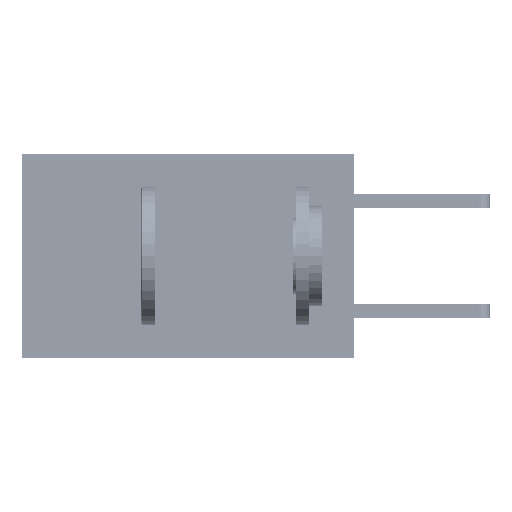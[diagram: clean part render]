
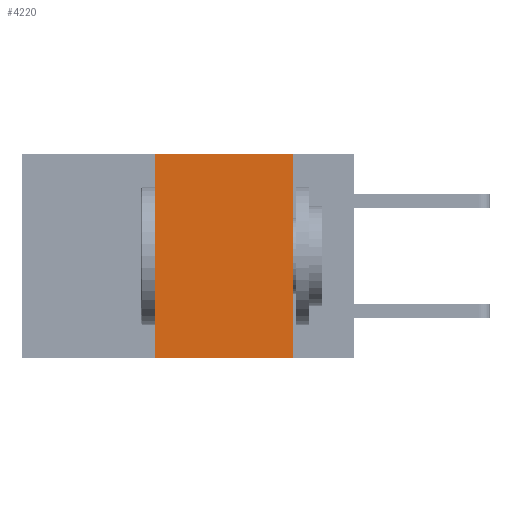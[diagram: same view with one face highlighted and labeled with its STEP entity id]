
A CAD part, left-side view. The second image highlights one B-rep face of the part: STEP entity #4220.
In plain terms, the highlighted planar face has unit normal (-1, 0, 0).
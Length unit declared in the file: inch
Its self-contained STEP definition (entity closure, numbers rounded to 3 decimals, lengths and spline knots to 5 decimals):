
#1895 = ORIENTED_EDGE ( 'NONE', *, *, #33448, .T. ) ;
#1991 = CARTESIAN_POINT ( 'NONE',  ( 0., 0.36, -0.37 ) ) ;
#4220 = ADVANCED_FACE ( 'NONE', ( #29030 ), #33040, .F. ) ;
#5551 = CARTESIAN_POINT ( 'NONE',  ( 0., 0.11, 0. ) ) ;
#6119 = DIRECTION ( 'NONE',  ( 0., -1., 0. ) ) ;
#8300 = CARTESIAN_POINT ( 'NONE',  ( 0., 0.6, 0. ) ) ;
#8950 = CARTESIAN_POINT ( 'NONE',  ( 0., 0.11, -0.37 ) ) ;
#9851 = DIRECTION ( 'NONE',  ( 1., 0., 0. ) ) ;
#11675 = CARTESIAN_POINT ( 'NONE',  ( 0., 0.6, -0.37 ) ) ;
#13910 = DIRECTION ( 'NONE',  ( 0., 0., 1. ) ) ;
#14808 = EDGE_CURVE ( 'NONE', #35982, #33792, #32213, .T. ) ;
#15068 = CARTESIAN_POINT ( 'NONE',  ( 0., 0.6, 0. ) ) ;
#15641 = EDGE_CURVE ( 'NONE', #33792, #22092, #30181, .T. ) ;
#15859 = LINE ( 'NONE', #25943, #37841 ) ;
#16263 = CARTESIAN_POINT ( 'NONE',  ( 0., 0.36, 0. ) ) ;
#17656 = ORIENTED_EDGE ( 'NONE', *, *, #15641, .F. ) ;
#17657 = DIRECTION ( 'NONE',  ( 0., -1., 0. ) ) ;
#18260 = VECTOR ( 'NONE', #24396, 39.37008 ) ;
#21992 = ORIENTED_EDGE ( 'NONE', *, *, #14808, .F. ) ;
#22092 = VERTEX_POINT ( 'NONE', #8950 ) ;
#23101 = VECTOR ( 'NONE', #6119, 39.37008 ) ;
#24396 = DIRECTION ( 'NONE',  ( 0., 0., -1. ) ) ;
#24484 = VECTOR ( 'NONE', #17657, 39.37008 ) ;
#25054 = DIRECTION ( 'NONE',  ( 0., 0., -1. ) ) ;
#25943 = CARTESIAN_POINT ( 'NONE',  ( 0., 0.36, 0. ) ) ;
#28069 = CARTESIAN_POINT ( 'NONE',  ( 0., 0.11, 0. ) ) ;
#29030 = FACE_OUTER_BOUND ( 'NONE', #32371, .T. ) ;
#29163 = VERTEX_POINT ( 'NONE', #1991 ) ;
#30181 = LINE ( 'NONE', #5551, #18260 ) ;
#32213 = LINE ( 'NONE', #15068, #23101 ) ;
#32371 = EDGE_LOOP ( 'NONE', ( #17656, #21992, #33578, #1895 ) ) ;
#33040 = PLANE ( 'NONE',  #33665 ) ;
#33448 = EDGE_CURVE ( 'NONE', #29163, #22092, #34515, .T. ) ;
#33578 = ORIENTED_EDGE ( 'NONE', *, *, #37401, .F. ) ;
#33665 = AXIS2_PLACEMENT_3D ( 'NONE', #8300, #9851, #25054 ) ;
#33792 = VERTEX_POINT ( 'NONE', #28069 ) ;
#34515 = LINE ( 'NONE', #11675, #24484 ) ;
#35982 = VERTEX_POINT ( 'NONE', #16263 ) ;
#37401 = EDGE_CURVE ( 'NONE', #29163, #35982, #15859, .T. ) ;
#37841 = VECTOR ( 'NONE', #13910, 39.37008 ) ;
